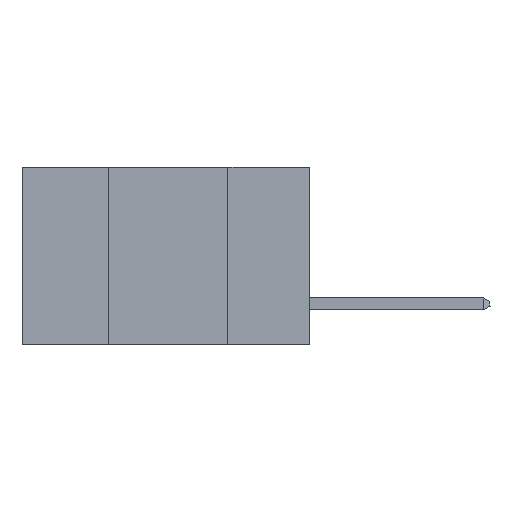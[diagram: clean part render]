
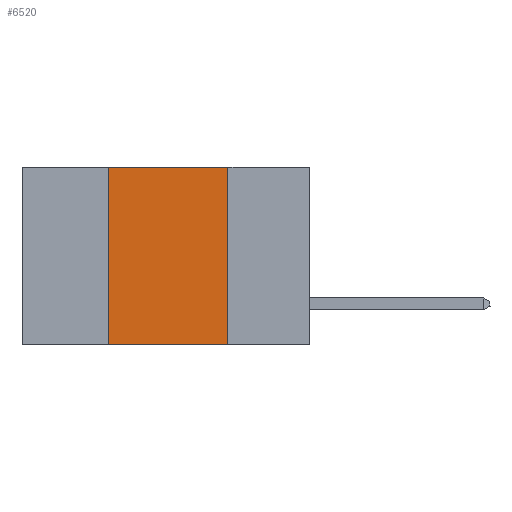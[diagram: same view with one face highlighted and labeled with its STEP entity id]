
A CAD part, left-side view. The second image highlights one B-rep face of the part: STEP entity #6520.
In plain terms, the highlighted planar face has unit normal (-1, 0, 0).
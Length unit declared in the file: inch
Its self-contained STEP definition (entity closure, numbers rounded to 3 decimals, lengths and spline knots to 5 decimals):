
#900 = CARTESIAN_POINT ( 'NONE',  ( 0., 0.42, 0. ) ) ;
#969 = CARTESIAN_POINT ( 'NONE',  ( 0., 0.6, 0. ) ) ;
#3696 = DIRECTION ( 'NONE',  ( 0., 0., -1. ) ) ;
#4092 = ORIENTED_EDGE ( 'NONE', *, *, #7799, .F. ) ;
#4378 = DIRECTION ( 'NONE',  ( 0., -1., 0. ) ) ;
#4575 = LINE ( 'NONE', #33097, #14462 ) ;
#5926 = AXIS2_PLACEMENT_3D ( 'NONE', #969, #10613, #3696 ) ;
#6520 = ADVANCED_FACE ( 'NONE', ( #26940 ), #39131, .F. ) ;
#6999 = EDGE_CURVE ( 'NONE', #17663, #32117, #37300, .T. ) ;
#7214 = CARTESIAN_POINT ( 'NONE',  ( 0., 0.6, 0. ) ) ;
#7799 = EDGE_CURVE ( 'NONE', #34315, #18593, #39336, .T. ) ;
#7887 = DIRECTION ( 'NONE',  ( 0., 0., 1. ) ) ;
#8172 = EDGE_CURVE ( 'NONE', #18593, #17663, #29653, .T. ) ;
#10613 = DIRECTION ( 'NONE',  ( 1., 0., 0. ) ) ;
#10623 = CARTESIAN_POINT ( 'NONE',  ( 0., 0.42, 0. ) ) ;
#12763 = EDGE_LOOP ( 'NONE', ( #15035, #35234, #4092, #16697 ) ) ;
#14462 = VECTOR ( 'NONE', #4378, 39.37008 ) ;
#15035 = ORIENTED_EDGE ( 'NONE', *, *, #6999, .F. ) ;
#15455 = VECTOR ( 'NONE', #33201, 39.37008 ) ;
#16129 = CARTESIAN_POINT ( 'NONE',  ( 0., 0.42, -0.37 ) ) ;
#16697 = ORIENTED_EDGE ( 'NONE', *, *, #27177, .T. ) ;
#17663 = VERTEX_POINT ( 'NONE', #19269 ) ;
#18593 = VERTEX_POINT ( 'NONE', #900 ) ;
#19269 = CARTESIAN_POINT ( 'NONE',  ( 0., 0.17, 0. ) ) ;
#24038 = VECTOR ( 'NONE', #31222, 39.37008 ) ;
#26940 = FACE_OUTER_BOUND ( 'NONE', #12763, .T. ) ;
#27177 = EDGE_CURVE ( 'NONE', #34315, #32117, #4575, .T. ) ;
#28131 = VECTOR ( 'NONE', #7887, 39.37008 ) ;
#29653 = LINE ( 'NONE', #7214, #15455 ) ;
#31222 = DIRECTION ( 'NONE',  ( 0., 0., -1. ) ) ;
#31434 = CARTESIAN_POINT ( 'NONE',  ( 0., 0.17, 0. ) ) ;
#32117 = VERTEX_POINT ( 'NONE', #36409 ) ;
#33097 = CARTESIAN_POINT ( 'NONE',  ( 0., 0.6, -0.37 ) ) ;
#33201 = DIRECTION ( 'NONE',  ( 0., -1., 0. ) ) ;
#34315 = VERTEX_POINT ( 'NONE', #16129 ) ;
#35234 = ORIENTED_EDGE ( 'NONE', *, *, #8172, .F. ) ;
#36409 = CARTESIAN_POINT ( 'NONE',  ( 0., 0.17, -0.37 ) ) ;
#37300 = LINE ( 'NONE', #31434, #24038 ) ;
#39131 = PLANE ( 'NONE',  #5926 ) ;
#39336 = LINE ( 'NONE', #10623, #28131 ) ;
